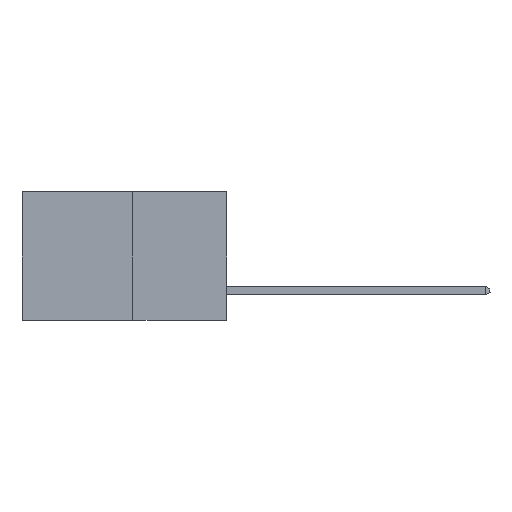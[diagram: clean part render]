
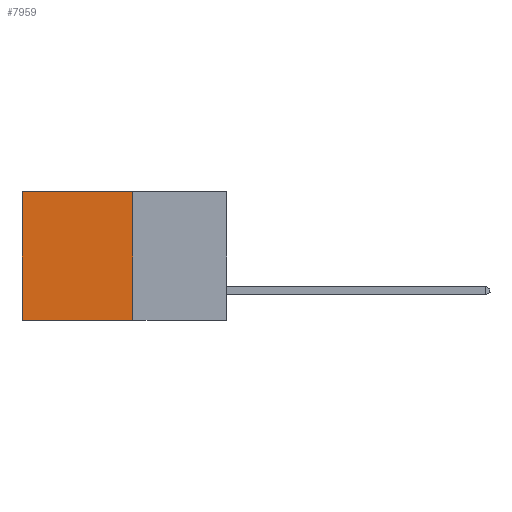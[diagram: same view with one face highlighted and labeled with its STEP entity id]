
A CAD part, left-side view. The second image highlights one B-rep face of the part: STEP entity #7959.
In plain terms, the highlighted planar face has unit normal (-1, 0, 0).
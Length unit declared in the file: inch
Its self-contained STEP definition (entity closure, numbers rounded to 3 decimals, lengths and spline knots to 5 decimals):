
#136 = VERTEX_POINT ( 'NONE', #15605 ) ;
#332 = VECTOR ( 'NONE', #29326, 39.37008 ) ;
#1215 = VECTOR ( 'NONE', #18394, 39.37008 ) ;
#1358 = PLANE ( 'NONE',  #27238 ) ;
#1967 = CARTESIAN_POINT ( 'NONE',  ( 0.277, 0.59, -0.37 ) ) ;
#2172 = EDGE_CURVE ( 'NONE', #136, #21054, #7652, .T. ) ;
#3276 = ORIENTED_EDGE ( 'NONE', *, *, #29986, .F. ) ;
#3789 = DIRECTION ( 'NONE',  ( 1., 0., 0. ) ) ;
#5366 = LINE ( 'NONE', #22510, #23878 ) ;
#5576 = DIRECTION ( 'NONE',  ( 0., 1., 0. ) ) ;
#7652 = LINE ( 'NONE', #28138, #1215 ) ;
#7959 = ADVANCED_FACE ( 'NONE', ( #16962 ), #1358, .F. ) ;
#8567 = CARTESIAN_POINT ( 'NONE',  ( 0.277, 0.27, -0.37 ) ) ;
#10067 = EDGE_CURVE ( 'NONE', #24886, #22142, #5366, .T. ) ;
#12791 = EDGE_CURVE ( 'NONE', #22142, #21054, #15072, .T. ) ;
#13700 = ORIENTED_EDGE ( 'NONE', *, *, #10067, .T. ) ;
#15072 = LINE ( 'NONE', #1967, #26238 ) ;
#15605 = CARTESIAN_POINT ( 'NONE',  ( 0.277, 0.27, -0.37 ) ) ;
#16535 = EDGE_LOOP ( 'NONE', ( #21785, #18156, #3276, #13700 ) ) ;
#16550 = DIRECTION ( 'NONE',  ( 0., 0., -1. ) ) ;
#16962 = FACE_OUTER_BOUND ( 'NONE', #16535, .T. ) ;
#18156 = ORIENTED_EDGE ( 'NONE', *, *, #2172, .F. ) ;
#18394 = DIRECTION ( 'NONE',  ( 0., 1., 0. ) ) ;
#18414 = CARTESIAN_POINT ( 'NONE',  ( 0.277, 0.27, 0. ) ) ;
#19655 = LINE ( 'NONE', #26965, #332 ) ;
#20738 = DIRECTION ( 'NONE',  ( 0., 0., -1. ) ) ;
#21054 = VERTEX_POINT ( 'NONE', #25699 ) ;
#21785 = ORIENTED_EDGE ( 'NONE', *, *, #12791, .T. ) ;
#22142 = VERTEX_POINT ( 'NONE', #27330 ) ;
#22510 = CARTESIAN_POINT ( 'NONE',  ( 0.277, 0.27, 0. ) ) ;
#23878 = VECTOR ( 'NONE', #5576, 39.37008 ) ;
#24886 = VERTEX_POINT ( 'NONE', #18414 ) ;
#25699 = CARTESIAN_POINT ( 'NONE',  ( 0.277, 0.59, -0.37 ) ) ;
#26238 = VECTOR ( 'NONE', #16550, 39.37008 ) ;
#26965 = CARTESIAN_POINT ( 'NONE',  ( 0.277, 0.27, -0.37 ) ) ;
#27238 = AXIS2_PLACEMENT_3D ( 'NONE', #8567, #3789, #20738 ) ;
#27330 = CARTESIAN_POINT ( 'NONE',  ( 0.277, 0.59, 0. ) ) ;
#28138 = CARTESIAN_POINT ( 'NONE',  ( 0.277, 0.27, -0.37 ) ) ;
#29326 = DIRECTION ( 'NONE',  ( 0., 0., -1. ) ) ;
#29986 = EDGE_CURVE ( 'NONE', #24886, #136, #19655, .T. ) ;
